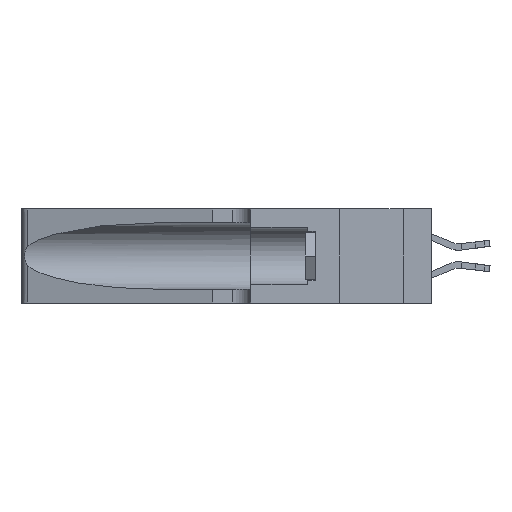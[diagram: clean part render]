
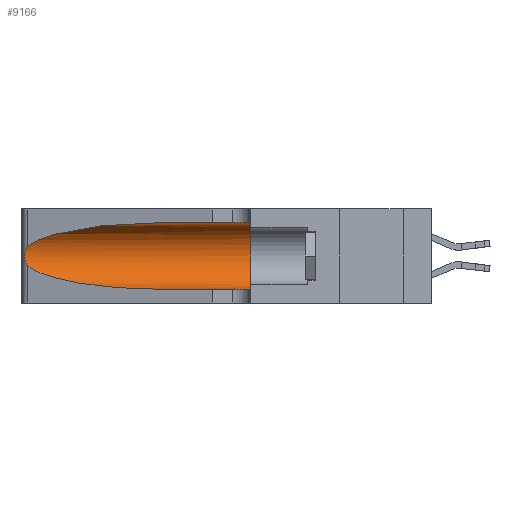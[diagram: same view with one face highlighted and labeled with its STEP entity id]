
A CAD part, left-side view. The second image highlights one B-rep face of the part: STEP entity #9166.
In plain terms, the highlighted cylindrical face has radius 3.308 mm (diameter 6.617 mm), a partial arc.
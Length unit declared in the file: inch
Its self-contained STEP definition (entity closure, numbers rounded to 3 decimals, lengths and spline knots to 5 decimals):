
#8 = CARTESIAN_POINT ( 'NONE',  ( 0.26018, 1.23835, 0.19895 ) ) ;
#298 = LINE ( 'NONE', #25953, #17903 ) ;
#640 = CARTESIAN_POINT ( 'NONE',  ( 0.25487, 1.22718, 0.22369 ) ) ;
#991 = CARTESIAN_POINT ( 'NONE',  ( 0.25487, 1.22718, 0.22369 ) ) ;
#1086 = VERTEX_POINT ( 'NONE', #25162 ) ;
#1298 = CARTESIAN_POINT ( 'NONE',  ( 0.2373, 1.15595, 0.28018 ) ) ;
#1851 = EDGE_CURVE ( 'NONE', #6876, #3402, #11644, .T. ) ;
#2749 = ORIENTED_EDGE ( 'NONE', *, *, #30342, .T. ) ;
#2929 = CARTESIAN_POINT ( 'NONE',  ( 0.25487, 1.22718, 0.14631 ) ) ;
#3388 = ORIENTED_EDGE ( 'NONE', *, *, #12958, .T. ) ;
#3402 = VERTEX_POINT ( 'NONE', #10961 ) ;
#3760 = DIRECTION ( 'NONE',  ( 0., -1., 0. ) ) ;
#4151 =( BOUNDED_CURVE ( )  B_SPLINE_CURVE ( 3, ( #2929, #19372, #21768, #21882 ),
 .UNSPECIFIED., .F., .T. ) 
 B_SPLINE_CURVE_WITH_KNOTS ( ( 4, 4 ),
 ( 3.44316, 4.71239 ),
 .UNSPECIFIED. ) 
 CURVE ( )  GEOMETRIC_REPRESENTATION_ITEM ( )  RATIONAL_B_SPLINE_CURVE ( ( 1., 0.87, 0.87, 1. ) ) 
 REPRESENTATION_ITEM ( '' )  );
#4323 = CARTESIAN_POINT ( 'NONE',  ( 0.1305, 0.72297, 0.05475 ) ) ;
#4891 = CARTESIAN_POINT ( 'NONE',  ( 0.25639, 1.23186, 0.15144 ) ) ;
#5469 = ORIENTED_EDGE ( 'NONE', *, *, #14993, .F. ) ;
#5698 = VERTEX_POINT ( 'NONE', #24831 ) ;
#5836 = CIRCLE ( 'NONE', #26412, 0.13025 ) ;
#5991 = CARTESIAN_POINT ( 'NONE',  ( 0.1305, 1.61858, 0.185 ) ) ;
#6499 = FACE_OUTER_BOUND ( 'NONE', #11362, .T. ) ;
#6876 = VERTEX_POINT ( 'NONE', #13225 ) ;
#7529 = CARTESIAN_POINT ( 'NONE',  ( 0.25555, 1.22993, 0.14849 ) ) ;
#7775 = ORIENTED_EDGE ( 'NONE', *, *, #9328, .T. ) ;
#8106 = CARTESIAN_POINT ( 'NONE',  ( 0.1305, 0.72297, 0.31525 ) ) ;
#9097 = CARTESIAN_POINT ( 'NONE',  ( 0.25639, 1.23184, 0.21858 ) ) ;
#9166 = ADVANCED_FACE ( 'NONE', ( #6499 ), #11742, .F. ) ;
#9328 = EDGE_CURVE ( 'NONE', #3402, #29057, #4151, .T. ) ;
#10347 = CARTESIAN_POINT ( 'NONE',  ( 0.1305, 0.35, 0.05475 ) ) ;
#10961 = CARTESIAN_POINT ( 'NONE',  ( 0.25487, 1.22718, 0.14631 ) ) ;
#11207 = VECTOR ( 'NONE', #18211, 39.37008 ) ;
#11362 = EDGE_LOOP ( 'NONE', ( #3388, #30721, #7775, #2749, #30449, #5469 ) ) ;
#11644 = B_SPLINE_CURVE_WITH_KNOTS ( 'NONE', 3,
 ( #640, #28097, #9097, #14233, #16831, #8, #23872, #21641, #22268, #24371, #26700, #4891, #7529, #12033 ),
 .UNSPECIFIED., .F., .F.,
 ( 4, 2, 2, 2, 2, 2, 4 ),
 ( 0., 0.00027, 0.00053, 0.00107, 0.0016, 0.00187, 0.00214 ),
 .UNSPECIFIED. ) ;
#11742 = CYLINDRICAL_SURFACE ( 'NONE', #12415, 0.13025 ) ;
#12033 = CARTESIAN_POINT ( 'NONE',  ( 0.25487, 1.22718, 0.14631 ) ) ;
#12207 =( BOUNDED_CURVE ( )  B_SPLINE_CURVE ( 3, ( #8106, #13235, #1298, #991 ),
 .UNSPECIFIED., .F., .T. ) 
 B_SPLINE_CURVE_WITH_KNOTS ( ( 4, 4 ),
 ( 1.5708, 2.84003 ),
 .UNSPECIFIED. ) 
 CURVE ( )  GEOMETRIC_REPRESENTATION_ITEM ( )  RATIONAL_B_SPLINE_CURVE ( ( 1., 0.87, 0.87, 1. ) ) 
 REPRESENTATION_ITEM ( '' )  );
#12415 = AXIS2_PLACEMENT_3D ( 'NONE', #5991, #3760, #15387 ) ;
#12958 = EDGE_CURVE ( 'NONE', #5698, #6876, #12207, .T. ) ;
#13204 = CARTESIAN_POINT ( 'NONE',  ( 0.1305, 1.61858, 0.05475 ) ) ;
#13225 = CARTESIAN_POINT ( 'NONE',  ( 0.25487, 1.22718, 0.22369 ) ) ;
#13235 = CARTESIAN_POINT ( 'NONE',  ( 0.18966, 0.96281, 0.31525 ) ) ;
#14233 = CARTESIAN_POINT ( 'NONE',  ( 0.25787, 1.23484, 0.2124 ) ) ;
#14993 = EDGE_CURVE ( 'NONE', #5698, #1086, #298, .T. ) ;
#15387 = DIRECTION ( 'NONE',  ( 0., 0., -1. ) ) ;
#16831 = CARTESIAN_POINT ( 'NONE',  ( 0.25854, 1.2359, 0.20912 ) ) ;
#17531 = LINE ( 'NONE', #13204, #11207 ) ;
#17903 = VECTOR ( 'NONE', #19222, 39.37008 ) ;
#18211 = DIRECTION ( 'NONE',  ( 0., -1., 0. ) ) ;
#19222 = DIRECTION ( 'NONE',  ( 0., -1., 0. ) ) ;
#19372 = CARTESIAN_POINT ( 'NONE',  ( 0.2373, 1.15595, 0.08982 ) ) ;
#20649 = VERTEX_POINT ( 'NONE', #10347 ) ;
#21641 = CARTESIAN_POINT ( 'NONE',  ( 0.26075, 1.23896, 0.178 ) ) ;
#21768 = CARTESIAN_POINT ( 'NONE',  ( 0.18966, 0.96281, 0.05475 ) ) ;
#21882 = CARTESIAN_POINT ( 'NONE',  ( 0.1305, 0.72297, 0.05475 ) ) ;
#22268 = CARTESIAN_POINT ( 'NONE',  ( 0.26017, 1.23833, 0.17102 ) ) ;
#23872 = CARTESIAN_POINT ( 'NONE',  ( 0.26075, 1.23896, 0.19203 ) ) ;
#24135 = DIRECTION ( 'NONE',  ( 0., 1., 0. ) ) ;
#24371 = CARTESIAN_POINT ( 'NONE',  ( 0.25856, 1.23593, 0.16098 ) ) ;
#24831 = CARTESIAN_POINT ( 'NONE',  ( 0.1305, 0.72297, 0.31525 ) ) ;
#25162 = CARTESIAN_POINT ( 'NONE',  ( 0.1305, 0.35, 0.31525 ) ) ;
#25410 = EDGE_CURVE ( 'NONE', #1086, #20649, #5836, .T. ) ;
#25953 = CARTESIAN_POINT ( 'NONE',  ( 0.1305, 1.61858, 0.31525 ) ) ;
#26149 = CARTESIAN_POINT ( 'NONE',  ( 0.1305, 0.35, 0.185 ) ) ;
#26412 = AXIS2_PLACEMENT_3D ( 'NONE', #26149, #24135, #26564 ) ;
#26564 = DIRECTION ( 'NONE',  ( 0., 0., 1. ) ) ;
#26700 = CARTESIAN_POINT ( 'NONE',  ( 0.25789, 1.23486, 0.15765 ) ) ;
#28097 = CARTESIAN_POINT ( 'NONE',  ( 0.25555, 1.22994, 0.2215 ) ) ;
#29057 = VERTEX_POINT ( 'NONE', #4323 ) ;
#30342 = EDGE_CURVE ( 'NONE', #29057, #20649, #17531, .T. ) ;
#30449 = ORIENTED_EDGE ( 'NONE', *, *, #25410, .F. ) ;
#30721 = ORIENTED_EDGE ( 'NONE', *, *, #1851, .T. ) ;
